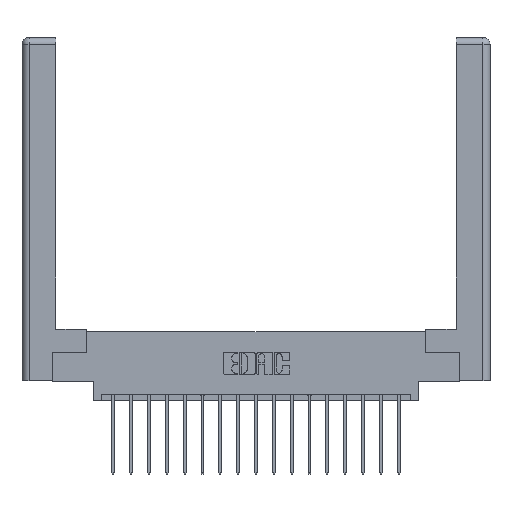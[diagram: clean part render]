
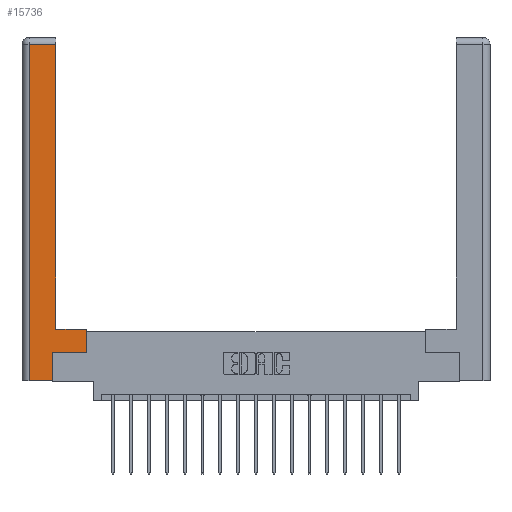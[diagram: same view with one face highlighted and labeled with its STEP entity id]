
A CAD part, top view. The second image highlights one B-rep face of the part: STEP entity #15736.
In plain terms, the highlighted planar face has unit normal (0, 0, 1).
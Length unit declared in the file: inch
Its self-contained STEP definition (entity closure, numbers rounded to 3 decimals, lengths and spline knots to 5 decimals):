
#472 = LINE ( 'NONE', #12946, #4167 ) ;
#533 = DIRECTION ( 'NONE',  ( 0., 1., 0. ) ) ;
#619 = VERTEX_POINT ( 'NONE', #5681 ) ;
#717 = DIRECTION ( 'NONE',  ( 1., 0., 0. ) ) ;
#766 = LINE ( 'NONE', #1098, #8430 ) ;
#878 = ORIENTED_EDGE ( 'NONE', *, *, #12719, .T. ) ;
#1098 = CARTESIAN_POINT ( 'NONE',  ( 0.295, 0.45, 0. ) ) ;
#1199 = VERTEX_POINT ( 'NONE', #9375 ) ;
#1214 = ORIENTED_EDGE ( 'NONE', *, *, #8705, .T. ) ;
#1315 = DIRECTION ( 'NONE',  ( 0., -1., 0. ) ) ;
#1535 = ORIENTED_EDGE ( 'NONE', *, *, #15677, .T. ) ;
#2077 = CARTESIAN_POINT ( 'NONE',  ( 0.265, 0.245, 0. ) ) ;
#2300 = VERTEX_POINT ( 'NONE', #12335 ) ;
#2604 = DIRECTION ( 'NONE',  ( -1., 0., 0. ) ) ;
#2773 = LINE ( 'NONE', #12748, #3234 ) ;
#2825 = CARTESIAN_POINT ( 'NONE',  ( 0.265, 0.245, 0. ) ) ;
#2892 = EDGE_CURVE ( 'NONE', #2300, #17058, #17329, .T. ) ;
#3234 = VECTOR ( 'NONE', #9730, 39.37008 ) ;
#3728 = CARTESIAN_POINT ( 'NONE',  ( 0.0615, 0., 0. ) ) ;
#3936 = EDGE_CURVE ( 'NONE', #7559, #2300, #12225, .T. ) ;
#3959 = DIRECTION ( 'NONE',  ( 1., 0., 0. ) ) ;
#3988 = CARTESIAN_POINT ( 'NONE',  ( 0.265, 0., 0. ) ) ;
#4167 = VECTOR ( 'NONE', #3959, 39.37008 ) ;
#4737 = VERTEX_POINT ( 'NONE', #3728 ) ;
#5061 = CARTESIAN_POINT ( 'NONE',  ( 0.295, 3., 0. ) ) ;
#5178 = CARTESIAN_POINT ( 'NONE',  ( 0.0615, 2.94, 0. ) ) ;
#5681 = CARTESIAN_POINT ( 'NONE',  ( 0.565, 0.245, 0. ) ) ;
#6067 = CARTESIAN_POINT ( 'NONE',  ( 0.295, 0.45, 0. ) ) ;
#6443 = CARTESIAN_POINT ( 'NONE',  ( 0.0615, 2.94, 0. ) ) ;
#6611 = EDGE_CURVE ( 'NONE', #17058, #4737, #17478, .T. ) ;
#6814 = DIRECTION ( 'NONE',  ( -1., 0., 0. ) ) ;
#7559 = VERTEX_POINT ( 'NONE', #6067 ) ;
#7785 = ORIENTED_EDGE ( 'NONE', *, *, #3936, .T. ) ;
#8430 = VECTOR ( 'NONE', #2604, 39.37008 ) ;
#8444 = CARTESIAN_POINT ( 'NONE',  ( 0., 0., 0. ) ) ;
#8705 = EDGE_CURVE ( 'NONE', #11668, #17926, #10173, .T. ) ;
#8805 = VECTOR ( 'NONE', #11132, 39.37008 ) ;
#9375 = CARTESIAN_POINT ( 'NONE',  ( 0.565, 0.45, 0. ) ) ;
#9592 = ORIENTED_EDGE ( 'NONE', *, *, #2892, .T. ) ;
#9730 = DIRECTION ( 'NONE',  ( 0., 1., 0. ) ) ;
#10155 = LINE ( 'NONE', #12154, #11809 ) ;
#10173 = LINE ( 'NONE', #2077, #8805 ) ;
#10504 = VECTOR ( 'NONE', #1315, 39.37008 ) ;
#11132 = DIRECTION ( 'NONE',  ( 0., 1., 0. ) ) ;
#11418 = DIRECTION ( 'NONE',  ( 0., 0., -1. ) ) ;
#11668 = VERTEX_POINT ( 'NONE', #3988 ) ;
#11809 = VECTOR ( 'NONE', #717, 39.37008 ) ;
#12154 = CARTESIAN_POINT ( 'NONE',  ( 0.265, 0., 0. ) ) ;
#12225 = LINE ( 'NONE', #5061, #12921 ) ;
#12335 = CARTESIAN_POINT ( 'NONE',  ( 0.295, 2.94, 0. ) ) ;
#12719 = EDGE_CURVE ( 'NONE', #1199, #7559, #766, .T. ) ;
#12748 = CARTESIAN_POINT ( 'NONE',  ( 0.565, 0.45, 0. ) ) ;
#12921 = VECTOR ( 'NONE', #533, 39.37008 ) ;
#12946 = CARTESIAN_POINT ( 'NONE',  ( 0.565, 0.245, 0. ) ) ;
#13053 = CARTESIAN_POINT ( 'NONE',  ( 0.0615, 0., 0. ) ) ;
#13062 = AXIS2_PLACEMENT_3D ( 'NONE', #8444, #11418, #6814 ) ;
#13418 = VECTOR ( 'NONE', #18463, 39.37008 ) ;
#13606 = ORIENTED_EDGE ( 'NONE', *, *, #14065, .T. ) ;
#14065 = EDGE_CURVE ( 'NONE', #17926, #619, #472, .T. ) ;
#14936 = ORIENTED_EDGE ( 'NONE', *, *, #6611, .T. ) ;
#15677 = EDGE_CURVE ( 'NONE', #619, #1199, #2773, .T. ) ;
#15736 = ADVANCED_FACE ( 'NONE', ( #18093 ), #18849, .F. ) ;
#15896 = EDGE_CURVE ( 'NONE', #4737, #11668, #10155, .T. ) ;
#16519 = EDGE_LOOP ( 'NONE', ( #7785, #9592, #14936, #17448, #1214, #13606, #1535, #878 ) ) ;
#17058 = VERTEX_POINT ( 'NONE', #6443 ) ;
#17329 = LINE ( 'NONE', #5178, #13418 ) ;
#17448 = ORIENTED_EDGE ( 'NONE', *, *, #15896, .T. ) ;
#17478 = LINE ( 'NONE', #13053, #10504 ) ;
#17926 = VERTEX_POINT ( 'NONE', #2825 ) ;
#18093 = FACE_OUTER_BOUND ( 'NONE', #16519, .T. ) ;
#18463 = DIRECTION ( 'NONE',  ( -1., 0., 0. ) ) ;
#18849 = PLANE ( 'NONE',  #13062 ) ;
